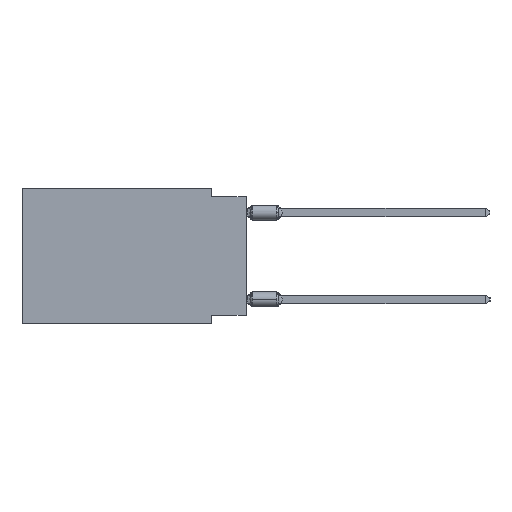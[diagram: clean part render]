
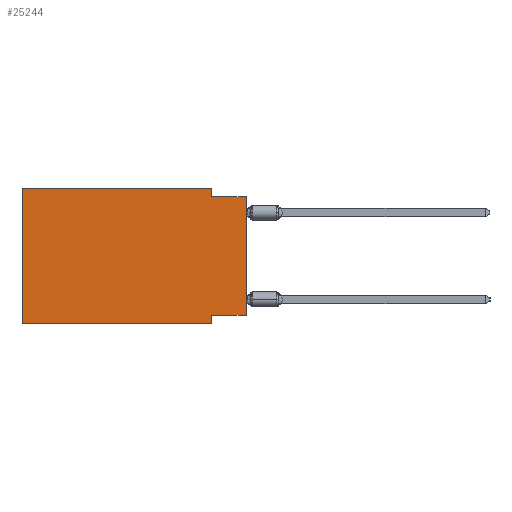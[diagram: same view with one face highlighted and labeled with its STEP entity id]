
A CAD part, left-side view. The second image highlights one B-rep face of the part: STEP entity #25244.
In plain terms, the highlighted planar face has unit normal (-1, 0, 0).
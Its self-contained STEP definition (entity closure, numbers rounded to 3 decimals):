
#592 = VERTEX_POINT ( 'NONE', #5751 ) ;
#609 = LINE ( 'NONE', #10708, #7591 ) ;
#699 = VECTOR ( 'NONE', #35361, 1000. ) ;
#711 = EDGE_CURVE ( 'NONE', #27952, #12208, #18842, .T. ) ;
#3497 = CARTESIAN_POINT ( 'NONE',  ( 0., 0., 0. ) ) ;
#4659 = LINE ( 'NONE', #33815, #22224 ) ;
#4730 = EDGE_CURVE ( 'NONE', #12208, #27385, #25810, .T. ) ;
#5485 = EDGE_CURVE ( 'NONE', #12177, #27952, #6188, .T. ) ;
#5751 = CARTESIAN_POINT ( 'NONE',  ( 0., 2.54, -9.271 ) ) ;
#5893 = LINE ( 'NONE', #3497, #24009 ) ;
#6080 = CARTESIAN_POINT ( 'NONE',  ( 0., 2.54, -9.906 ) ) ;
#6188 = LINE ( 'NONE', #22286, #699 ) ;
#7591 = VECTOR ( 'NONE', #23156, 1000. ) ;
#8084 = ORIENTED_EDGE ( 'NONE', *, *, #15397, .T. ) ;
#8436 = ORIENTED_EDGE ( 'NONE', *, *, #5485, .F. ) ;
#8537 = CARTESIAN_POINT ( 'NONE',  ( 0., 16.383, 0. ) ) ;
#8982 = ORIENTED_EDGE ( 'NONE', *, *, #33571, .F. ) ;
#9395 = VECTOR ( 'NONE', #41686, 1000. ) ;
#9521 = DIRECTION ( 'NONE',  ( 0., 0., 1. ) ) ;
#10708 = CARTESIAN_POINT ( 'NONE',  ( 0., 16.383, -9.906 ) ) ;
#11914 = ORIENTED_EDGE ( 'NONE', *, *, #22345, .T. ) ;
#12177 = VERTEX_POINT ( 'NONE', #15466 ) ;
#12208 = VERTEX_POINT ( 'NONE', #25318 ) ;
#12392 = DIRECTION ( 'NONE',  ( 0., 0., -1. ) ) ;
#12514 = DIRECTION ( 'NONE',  ( 0., 0., -1. ) ) ;
#14054 = CARTESIAN_POINT ( 'NONE',  ( 0., 16.383, -9.906 ) ) ;
#14808 = CARTESIAN_POINT ( 'NONE',  ( 0., 2.54, -9.906 ) ) ;
#15397 = EDGE_CURVE ( 'NONE', #19185, #27385, #5893, .T. ) ;
#15466 = CARTESIAN_POINT ( 'NONE',  ( 0., 16.383, 0. ) ) ;
#15617 = PLANE ( 'NONE',  #28646 ) ;
#15749 = DIRECTION ( 'NONE',  ( 0., -1., 0. ) ) ;
#18842 = LINE ( 'NONE', #22257, #21419 ) ;
#19185 = VERTEX_POINT ( 'NONE', #25274 ) ;
#20527 = DIRECTION ( 'NONE',  ( 0., 0., 1. ) ) ;
#21419 = VECTOR ( 'NONE', #35334, 1000. ) ;
#21521 = EDGE_LOOP ( 'NONE', ( #8084, #21719, #26147, #8436, #32400, #11914, #40046, #8982 ) ) ;
#21719 = ORIENTED_EDGE ( 'NONE', *, *, #4730, .F. ) ;
#22224 = VECTOR ( 'NONE', #20527, 1000. ) ;
#22257 = CARTESIAN_POINT ( 'NONE',  ( 0., 2.54, 0. ) ) ;
#22286 = CARTESIAN_POINT ( 'NONE',  ( 0., 16.383, 0. ) ) ;
#22345 = EDGE_CURVE ( 'NONE', #41830, #37416, #609, .T. ) ;
#23156 = DIRECTION ( 'NONE',  ( 0., -1., 0. ) ) ;
#23430 = EDGE_CURVE ( 'NONE', #592, #37416, #38668, .T. ) ;
#24009 = VECTOR ( 'NONE', #9521, 1000. ) ;
#24761 = LINE ( 'NONE', #28830, #9395 ) ;
#25244 = ADVANCED_FACE ( 'NONE', ( #32328 ), #15617, .F. ) ;
#25274 = CARTESIAN_POINT ( 'NONE',  ( 0., 0., -9.271 ) ) ;
#25318 = CARTESIAN_POINT ( 'NONE',  ( 0., 2.54, -0.635 ) ) ;
#25389 = VECTOR ( 'NONE', #12514, 1000. ) ;
#25810 = LINE ( 'NONE', #32056, #30813 ) ;
#26147 = ORIENTED_EDGE ( 'NONE', *, *, #711, .F. ) ;
#27385 = VERTEX_POINT ( 'NONE', #30210 ) ;
#27952 = VERTEX_POINT ( 'NONE', #30158 ) ;
#28646 = AXIS2_PLACEMENT_3D ( 'NONE', #8537, #42185, #12392 ) ;
#28830 = CARTESIAN_POINT ( 'NONE',  ( 0., 0., -9.271 ) ) ;
#30158 = CARTESIAN_POINT ( 'NONE',  ( 0., 2.54, 0. ) ) ;
#30189 = EDGE_CURVE ( 'NONE', #41830, #12177, #4659, .T. ) ;
#30210 = CARTESIAN_POINT ( 'NONE',  ( 0., 0., -0.635 ) ) ;
#30813 = VECTOR ( 'NONE', #15749, 1000. ) ;
#32056 = CARTESIAN_POINT ( 'NONE',  ( 0., 0., -0.635 ) ) ;
#32328 = FACE_OUTER_BOUND ( 'NONE', #21521, .T. ) ;
#32400 = ORIENTED_EDGE ( 'NONE', *, *, #30189, .F. ) ;
#33571 = EDGE_CURVE ( 'NONE', #19185, #592, #24761, .T. ) ;
#33815 = CARTESIAN_POINT ( 'NONE',  ( 0., 16.383, 0. ) ) ;
#35334 = DIRECTION ( 'NONE',  ( 0., 0., -1. ) ) ;
#35361 = DIRECTION ( 'NONE',  ( 0., -1., 0. ) ) ;
#37416 = VERTEX_POINT ( 'NONE', #14808 ) ;
#38668 = LINE ( 'NONE', #6080, #25389 ) ;
#40046 = ORIENTED_EDGE ( 'NONE', *, *, #23430, .F. ) ;
#41686 = DIRECTION ( 'NONE',  ( 0., 1., 0. ) ) ;
#41830 = VERTEX_POINT ( 'NONE', #14054 ) ;
#42185 = DIRECTION ( 'NONE',  ( 1., 0., 0. ) ) ;
